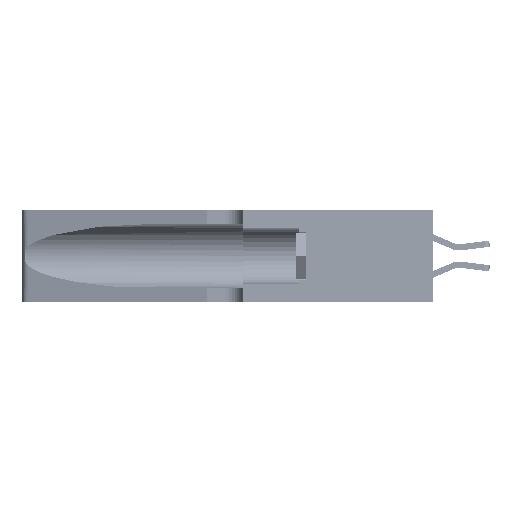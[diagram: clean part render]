
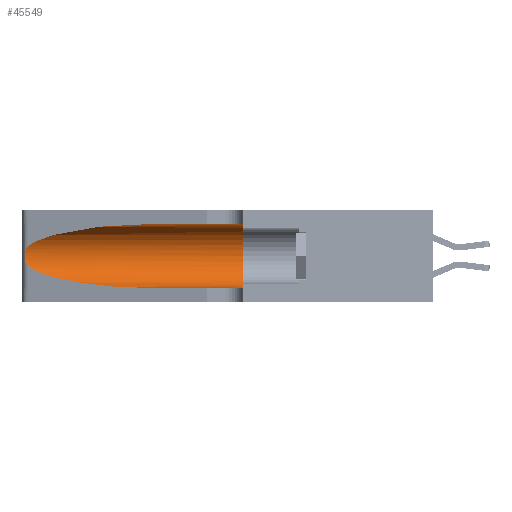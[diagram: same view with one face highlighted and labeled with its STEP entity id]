
A CAD part, left-side view. The second image highlights one B-rep face of the part: STEP entity #45549.
In plain terms, the highlighted cylindrical face has radius 3.308 mm (diameter 6.617 mm), a partial arc.
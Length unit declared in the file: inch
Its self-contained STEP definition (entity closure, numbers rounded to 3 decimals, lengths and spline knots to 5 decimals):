
#332 =( BOUNDED_CURVE ( )  B_SPLINE_CURVE ( 3, ( #30746, #2311, #42964, #18755 ),
 .UNSPECIFIED., .F., .F. ) 
 B_SPLINE_CURVE_WITH_KNOTS ( ( 4, 4 ),
 ( 3.44316, 4.71239 ),
 .UNSPECIFIED. ) 
 CURVE ( )  GEOMETRIC_REPRESENTATION_ITEM ( )  RATIONAL_B_SPLINE_CURVE ( ( 1., 0.87, 0.87, 1. ) ) 
 REPRESENTATION_ITEM ( '' )  );
#429 = CIRCLE ( 'NONE', #22068, 0.13025 ) ;
#1106 = CARTESIAN_POINT ( 'NONE',  ( 0.25639, 1.23184, 0.21858 ) ) ;
#1276 = CARTESIAN_POINT ( 'NONE',  ( 0.25639, 1.23186, 0.15144 ) ) ;
#1859 = DIRECTION ( 'NONE',  ( 0., 1., 0. ) ) ;
#2311 = CARTESIAN_POINT ( 'NONE',  ( 0.2373, 1.15595, 0.08982 ) ) ;
#5146 = CARTESIAN_POINT ( 'NONE',  ( 0.1305, 0.72297, 0.05475 ) ) ;
#5390 = CARTESIAN_POINT ( 'NONE',  ( 0.25487, 1.22718, 0.14631 ) ) ;
#7516 = CARTESIAN_POINT ( 'NONE',  ( 0.18966, 0.96281, 0.31525 ) ) ;
#9336 = CARTESIAN_POINT ( 'NONE',  ( 0.25487, 1.22718, 0.22369 ) ) ;
#10864 = CARTESIAN_POINT ( 'NONE',  ( 0.25487, 1.22718, 0.22369 ) ) ;
#11103 = ORIENTED_EDGE ( 'NONE', *, *, #38986, .T. ) ;
#11259 = LINE ( 'NONE', #43936, #20801 ) ;
#11571 = DIRECTION ( 'NONE',  ( 0., -1., 0. ) ) ;
#11658 = CARTESIAN_POINT ( 'NONE',  ( 0.2373, 1.15595, 0.28018 ) ) ;
#12873 = VERTEX_POINT ( 'NONE', #27118 ) ;
#13464 = CARTESIAN_POINT ( 'NONE',  ( 0.25854, 1.2359, 0.20912 ) ) ;
#16154 = AXIS2_PLACEMENT_3D ( 'NONE', #22749, #50940, #18669 ) ;
#17208 = FACE_OUTER_BOUND ( 'NONE', #45690, .T. ) ;
#17565 = CARTESIAN_POINT ( 'NONE',  ( 0.26075, 1.23896, 0.19203 ) ) ;
#17669 = VERTEX_POINT ( 'NONE', #38617 ) ;
#18669 = DIRECTION ( 'NONE',  ( 0., 0., -1. ) ) ;
#18755 = CARTESIAN_POINT ( 'NONE',  ( 0.1305, 0.72297, 0.05475 ) ) ;
#19184 = EDGE_CURVE ( 'NONE', #24428, #21203, #11259, .T. ) ;
#20801 = VECTOR ( 'NONE', #11571, 39.37008 ) ;
#21203 = VERTEX_POINT ( 'NONE', #38304 ) ;
#21632 = CARTESIAN_POINT ( 'NONE',  ( 0.26017, 1.23833, 0.17102 ) ) ;
#22068 = AXIS2_PLACEMENT_3D ( 'NONE', #26227, #1859, #30301 ) ;
#22749 = CARTESIAN_POINT ( 'NONE',  ( 0.1305, 1.61858, 0.185 ) ) ;
#23257 = B_SPLINE_CURVE_WITH_KNOTS ( 'NONE', 3,
 ( #9336, #33625, #1106, #37710, #13464, #41772, #17565, #45804, #21632, #49854, #25677, #1276, #29733, #5390 ),
 .UNSPECIFIED., .F., .F.,
 ( 4, 2, 2, 2, 2, 2, 4 ),
 ( 0., 0.00027, 0.00053, 0.00107, 0.0016, 0.00187, 0.00214 ),
 .UNSPECIFIED. ) ;
#23815 = EDGE_CURVE ( 'NONE', #35909, #42642, #23257, .T. ) ;
#24428 = VERTEX_POINT ( 'NONE', #5146 ) ;
#24465 = ORIENTED_EDGE ( 'NONE', *, *, #23815, .T. ) ;
#25677 = CARTESIAN_POINT ( 'NONE',  ( 0.25789, 1.23486, 0.15765 ) ) ;
#26227 = CARTESIAN_POINT ( 'NONE',  ( 0.1305, 0.35, 0.185 ) ) ;
#26677 = CYLINDRICAL_SURFACE ( 'NONE', #16154, 0.13025 ) ;
#27118 = CARTESIAN_POINT ( 'NONE',  ( 0.1305, 0.35, 0.31525 ) ) ;
#29733 = CARTESIAN_POINT ( 'NONE',  ( 0.25555, 1.22993, 0.14849 ) ) ;
#30301 = DIRECTION ( 'NONE',  ( 0., 0., 1. ) ) ;
#30746 = CARTESIAN_POINT ( 'NONE',  ( 0.25487, 1.22718, 0.14631 ) ) ;
#31342 = EDGE_CURVE ( 'NONE', #17669, #35909, #47502, .T. ) ;
#31828 = CARTESIAN_POINT ( 'NONE',  ( 0.1305, 0.72297, 0.31525 ) ) ;
#33625 = CARTESIAN_POINT ( 'NONE',  ( 0.25555, 1.22994, 0.2215 ) ) ;
#35116 = DIRECTION ( 'NONE',  ( 0., -1., 0. ) ) ;
#35909 = VERTEX_POINT ( 'NONE', #10864 ) ;
#35919 = VECTOR ( 'NONE', #35116, 39.37008 ) ;
#36418 = EDGE_CURVE ( 'NONE', #12873, #21203, #429, .T. ) ;
#37710 = CARTESIAN_POINT ( 'NONE',  ( 0.25787, 1.23484, 0.2124 ) ) ;
#38304 = CARTESIAN_POINT ( 'NONE',  ( 0.1305, 0.35, 0.05475 ) ) ;
#38617 = CARTESIAN_POINT ( 'NONE',  ( 0.1305, 0.72297, 0.31525 ) ) ;
#38986 = EDGE_CURVE ( 'NONE', #42642, #24428, #332, .T. ) ;
#39978 = CARTESIAN_POINT ( 'NONE',  ( 0.25487, 1.22718, 0.22369 ) ) ;
#41599 = EDGE_CURVE ( 'NONE', #17669, #12873, #46655, .T. ) ;
#41772 = CARTESIAN_POINT ( 'NONE',  ( 0.26018, 1.23835, 0.19895 ) ) ;
#42642 = VERTEX_POINT ( 'NONE', #47856 ) ;
#42964 = CARTESIAN_POINT ( 'NONE',  ( 0.18966, 0.96281, 0.05475 ) ) ;
#43936 = CARTESIAN_POINT ( 'NONE',  ( 0.1305, 1.61858, 0.05475 ) ) ;
#44739 = ORIENTED_EDGE ( 'NONE', *, *, #36418, .F. ) ;
#45432 = ORIENTED_EDGE ( 'NONE', *, *, #31342, .T. ) ;
#45549 = ADVANCED_FACE ( 'NONE', ( #17208 ), #26677, .F. ) ;
#45690 = EDGE_LOOP ( 'NONE', ( #45432, #24465, #11103, #50458, #44739, #50923 ) ) ;
#45804 = CARTESIAN_POINT ( 'NONE',  ( 0.26075, 1.23896, 0.178 ) ) ;
#46655 = LINE ( 'NONE', #51155, #35919 ) ;
#47502 =( BOUNDED_CURVE ( )  B_SPLINE_CURVE ( 3, ( #31828, #7516, #11658, #39978 ),
 .UNSPECIFIED., .F., .F. ) 
 B_SPLINE_CURVE_WITH_KNOTS ( ( 4, 4 ),
 ( 1.5708, 2.84003 ),
 .UNSPECIFIED. ) 
 CURVE ( )  GEOMETRIC_REPRESENTATION_ITEM ( )  RATIONAL_B_SPLINE_CURVE ( ( 1., 0.87, 0.87, 1. ) ) 
 REPRESENTATION_ITEM ( '' )  );
#47856 = CARTESIAN_POINT ( 'NONE',  ( 0.25487, 1.22718, 0.14631 ) ) ;
#49854 = CARTESIAN_POINT ( 'NONE',  ( 0.25856, 1.23593, 0.16098 ) ) ;
#50458 = ORIENTED_EDGE ( 'NONE', *, *, #19184, .T. ) ;
#50923 = ORIENTED_EDGE ( 'NONE', *, *, #41599, .F. ) ;
#50940 = DIRECTION ( 'NONE',  ( 0., -1., 0. ) ) ;
#51155 = CARTESIAN_POINT ( 'NONE',  ( 0.1305, 1.61858, 0.31525 ) ) ;
